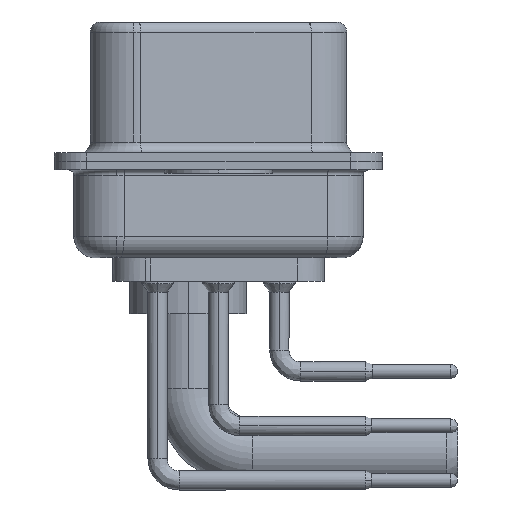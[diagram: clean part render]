
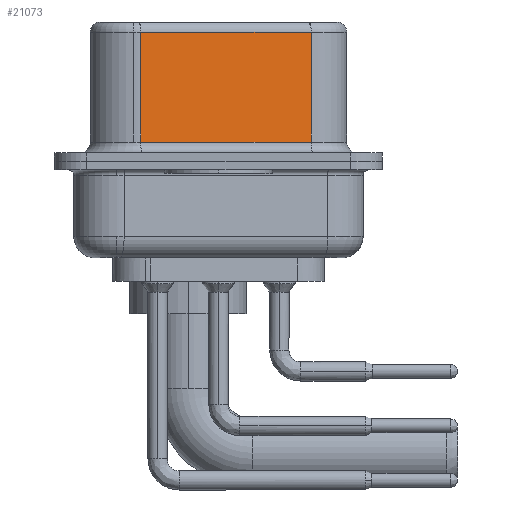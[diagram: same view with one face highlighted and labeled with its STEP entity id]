
A CAD part, left-side view. The second image highlights one B-rep face of the part: STEP entity #21073.
In plain terms, the highlighted planar face has unit normal (-0.985, -0.174, 0).
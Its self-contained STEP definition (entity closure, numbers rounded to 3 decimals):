
#1339 = VECTOR ( 'NONE', #7117, 1000. ) ;
#1402 = EDGE_CURVE ( 'NONE', #9571, #23883, #7804, .T. ) ;
#1586 = DIRECTION ( 'NONE',  ( 0., 0., -1. ) ) ;
#1753 = PLANE ( 'NONE',  #8330 ) ;
#2502 = CARTESIAN_POINT ( 'NONE',  ( 3.73, 3.628, 0.9 ) ) ;
#3271 = VECTOR ( 'NONE', #32127, 1000. ) ;
#3299 = CARTESIAN_POINT ( 'NONE',  ( 5.132, -4.322, 0.9 ) ) ;
#3666 = VERTEX_POINT ( 'NONE', #2502 ) ;
#3824 = ORIENTED_EDGE ( 'NONE', *, *, #27276, .F. ) ;
#5100 = CARTESIAN_POINT ( 'NONE',  ( 5.132, -4.322, 6.02 ) ) ;
#7117 = DIRECTION ( 'NONE',  ( 0.174, -0.985, 0. ) ) ;
#7804 = LINE ( 'NONE', #18242, #3271 ) ;
#7999 = EDGE_CURVE ( 'NONE', #23883, #3666, #31488, .T. ) ;
#8330 = AXIS2_PLACEMENT_3D ( 'NONE', #12730, #34166, #23701 ) ;
#9276 = CARTESIAN_POINT ( 'NONE',  ( 5.132, -4.322, 0.9 ) ) ;
#9571 = VERTEX_POINT ( 'NONE', #5100 ) ;
#10727 = EDGE_CURVE ( 'NONE', #3666, #18766, #20242, .T. ) ;
#11755 = ORIENTED_EDGE ( 'NONE', *, *, #7999, .T. ) ;
#12730 = CARTESIAN_POINT ( 'NONE',  ( 5.132, -4.322, 6.52 ) ) ;
#13460 = LINE ( 'NONE', #16330, #31293 ) ;
#15427 = CARTESIAN_POINT ( 'NONE',  ( 3.73, 3.628, 6.52 ) ) ;
#16330 = CARTESIAN_POINT ( 'NONE',  ( 5.132, -4.322, 6.52 ) ) ;
#17765 = EDGE_LOOP ( 'NONE', ( #3824, #26154, #11755, #17947 ) ) ;
#17947 = ORIENTED_EDGE ( 'NONE', *, *, #10727, .T. ) ;
#18242 = CARTESIAN_POINT ( 'NONE',  ( 5.132, -4.322, 6.02 ) ) ;
#18766 = VERTEX_POINT ( 'NONE', #3299 ) ;
#20242 = LINE ( 'NONE', #9276, #1339 ) ;
#21073 = ADVANCED_FACE ( 'NONE', ( #31486 ), #1753, .F. ) ;
#22489 = VECTOR ( 'NONE', #1586, 1000. ) ;
#23701 = DIRECTION ( 'NONE',  ( -0.174, 0.985, 0. ) ) ;
#23883 = VERTEX_POINT ( 'NONE', #34762 ) ;
#26154 = ORIENTED_EDGE ( 'NONE', *, *, #1402, .T. ) ;
#27276 = EDGE_CURVE ( 'NONE', #9571, #18766, #13460, .T. ) ;
#27348 = DIRECTION ( 'NONE',  ( 0., 0., -1. ) ) ;
#31293 = VECTOR ( 'NONE', #27348, 1000. ) ;
#31486 = FACE_OUTER_BOUND ( 'NONE', #17765, .T. ) ;
#31488 = LINE ( 'NONE', #15427, #22489 ) ;
#32127 = DIRECTION ( 'NONE',  ( -0.174, 0.985, 0. ) ) ;
#34166 = DIRECTION ( 'NONE',  ( 0.985, 0.174, 0. ) ) ;
#34762 = CARTESIAN_POINT ( 'NONE',  ( 3.73, 3.628, 6.02 ) ) ;
